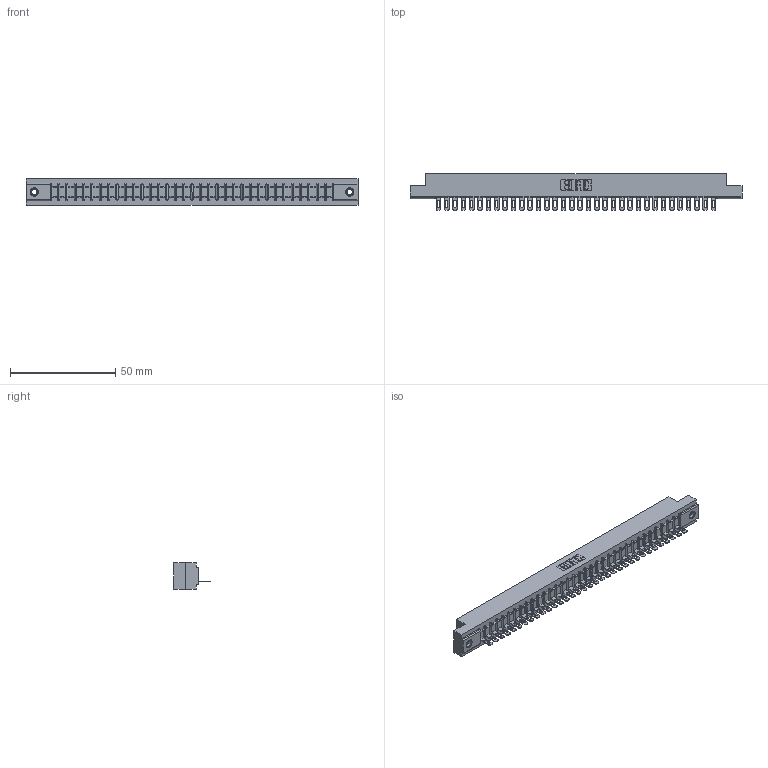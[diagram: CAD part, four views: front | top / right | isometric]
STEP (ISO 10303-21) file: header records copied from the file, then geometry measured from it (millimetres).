
FILE_DESCRIPTION (( 'STEP AP203' ), '1' );
FILE_NAME ('307-034-501-107.STEP', '2019-09-05T06:21:47', ( '' ), ( '' ), 'SwSTEP 2.0', 'SolidWorks 2016', '' );
FILE_SCHEMA (( 'CONFIG_CONTROL_DESIGN' ));
Length unit declared in the file: inch
Products named in the file (4): 345-250-001_345-250-005-103; 307 Part_.156 Dia Mounting Holes; 307-034-501-107; 307-290-002_501
Assembly tree (37 placements, depth 2):
  307-034-501-107
    307 Part_.156 Dia Mounting Holes
    307-290-002_501  x34
    345-250-001_345-250-005-103  x2
Bounding box: 157.73 x 17.42 x 12.7 mm (x, y, z)
Volume: 16836 mm3; surface area: 21255.9 mm2
Topology: 37 solids, 37 shells, 2797 faces, 8551 edges, 5598 vertices
Faces by surface type: plane 1598, cylinder 1113, sphere 70, cone 12, torus 4
Entity records: 32113 total; most frequent: CARTESIAN_POINT 5395, ORIENTED_EDGE 5378, DIRECTION 5259, EDGE_CURVE 2689, LINE 2051, VECTOR 2051, VERTEX_POINT 1740, AXIS2_PLACEMENT_3D 1604
